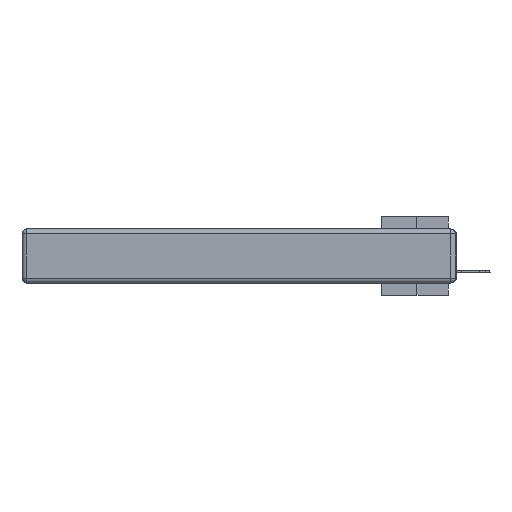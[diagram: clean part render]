
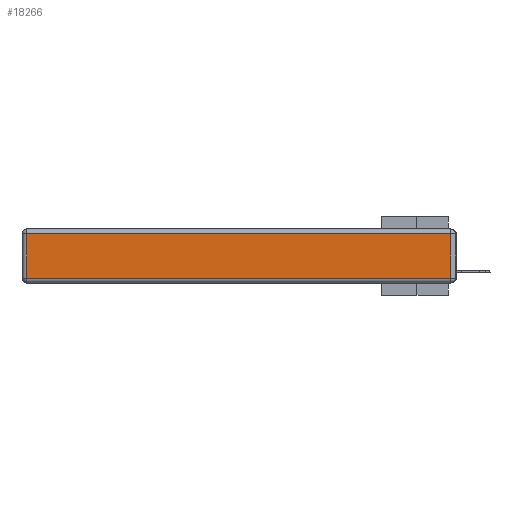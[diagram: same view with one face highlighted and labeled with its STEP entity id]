
A CAD part, left-side view. The second image highlights one B-rep face of the part: STEP entity #18266.
In plain terms, the highlighted planar face has unit normal (-1, 0, 0).
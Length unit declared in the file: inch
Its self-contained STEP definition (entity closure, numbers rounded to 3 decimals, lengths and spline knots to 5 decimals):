
#390 = CARTESIAN_POINT ( 'NONE',  ( 0., 2.72, -0.313 ) ) ;
#1413 = VECTOR ( 'NONE', #32704, 39.37008 ) ;
#2040 = ORIENTED_EDGE ( 'NONE', *, *, #6627, .T. ) ;
#5474 = PLANE ( 'NONE',  #20604 ) ;
#6627 = EDGE_CURVE ( 'NONE', #7891, #25221, #19716, .T. ) ;
#7161 = CARTESIAN_POINT ( 'NONE',  ( 0., 2.75, -0.03 ) ) ;
#7445 = CARTESIAN_POINT ( 'NONE',  ( 0., 0., -0.343 ) ) ;
#7891 = VERTEX_POINT ( 'NONE', #390 ) ;
#7946 = CARTESIAN_POINT ( 'NONE',  ( 0., 0.03, -0.03 ) ) ;
#9156 = EDGE_CURVE ( 'NONE', #25221, #10296, #30083, .T. ) ;
#9686 = ORIENTED_EDGE ( 'NONE', *, *, #32997, .T. ) ;
#10296 = VERTEX_POINT ( 'NONE', #7946 ) ;
#12713 = LINE ( 'NONE', #7161, #26604 ) ;
#13769 = ORIENTED_EDGE ( 'NONE', *, *, #9156, .T. ) ;
#14154 = CARTESIAN_POINT ( 'NONE',  ( 0., 0., -0.313 ) ) ;
#14671 = VERTEX_POINT ( 'NONE', #30852 ) ;
#15215 = ORIENTED_EDGE ( 'NONE', *, *, #22164, .T. ) ;
#16754 = DIRECTION ( 'NONE',  ( 0., -1., 0. ) ) ;
#18266 = ADVANCED_FACE ( 'NONE', ( #30841 ), #5474, .T. ) ;
#18471 = DIRECTION ( 'NONE',  ( 0., 1., 0. ) ) ;
#19106 = CARTESIAN_POINT ( 'NONE',  ( 0., 0.03, -0.313 ) ) ;
#19716 = LINE ( 'NONE', #14154, #33567 ) ;
#20604 = AXIS2_PLACEMENT_3D ( 'NONE', #7445, #21354, #24491 ) ;
#21354 = DIRECTION ( 'NONE',  ( -1., 0., 0. ) ) ;
#21953 = CARTESIAN_POINT ( 'NONE',  ( 0., 0.03, -0.343 ) ) ;
#22164 = EDGE_CURVE ( 'NONE', #14671, #7891, #35815, .T. ) ;
#24491 = DIRECTION ( 'NONE',  ( 0., 0., 1. ) ) ;
#25221 = VERTEX_POINT ( 'NONE', #19106 ) ;
#26604 = VECTOR ( 'NONE', #18471, 39.37008 ) ;
#29300 = VECTOR ( 'NONE', #29723, 39.37008 ) ;
#29535 = EDGE_LOOP ( 'NONE', ( #2040, #13769, #9686, #15215 ) ) ;
#29723 = DIRECTION ( 'NONE',  ( 0., 0., 1. ) ) ;
#30083 = LINE ( 'NONE', #21953, #29300 ) ;
#30841 = FACE_OUTER_BOUND ( 'NONE', #29535, .T. ) ;
#30852 = CARTESIAN_POINT ( 'NONE',  ( 0., 2.72, -0.03 ) ) ;
#32704 = DIRECTION ( 'NONE',  ( 0., 0., -1. ) ) ;
#32997 = EDGE_CURVE ( 'NONE', #10296, #14671, #12713, .T. ) ;
#33254 = CARTESIAN_POINT ( 'NONE',  ( 0., 2.72, -0.343 ) ) ;
#33567 = VECTOR ( 'NONE', #16754, 39.37008 ) ;
#35815 = LINE ( 'NONE', #33254, #1413 ) ;
